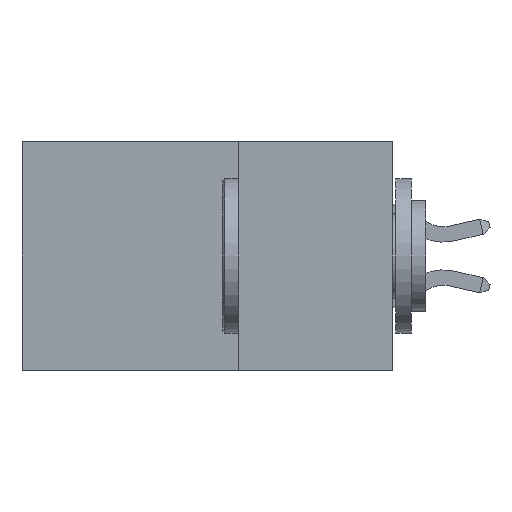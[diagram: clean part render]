
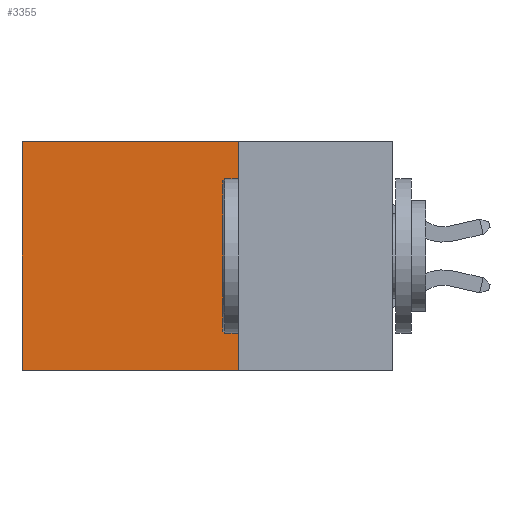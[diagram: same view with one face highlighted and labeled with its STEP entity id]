
A CAD part, left-side view. The second image highlights one B-rep face of the part: STEP entity #3355.
In plain terms, the highlighted planar face has unit normal (-1, 0, 0).
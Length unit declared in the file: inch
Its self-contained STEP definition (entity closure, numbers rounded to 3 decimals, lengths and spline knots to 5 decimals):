
#85 = CARTESIAN_POINT ( 'NONE',  ( 0.2875, 0.6, 0. ) ) ;
#1599 = DIRECTION ( 'NONE',  ( 0., 0., -1. ) ) ;
#1624 = DIRECTION ( 'NONE',  ( 1., 0., 0. ) ) ;
#1692 = CARTESIAN_POINT ( 'NONE',  ( 0.2875, 0.25, 0. ) ) ;
#2339 = VECTOR ( 'NONE', #8807, 39.37008 ) ;
#2370 = PLANE ( 'NONE',  #23709 ) ;
#3038 = LINE ( 'NONE', #85, #2339 ) ;
#3355 = ADVANCED_FACE ( 'NONE', ( #17948 ), #2370, .F. ) ;
#3544 = VERTEX_POINT ( 'NONE', #26406 ) ;
#4168 = EDGE_CURVE ( 'NONE', #6374, #3544, #4899, .T. ) ;
#4899 = LINE ( 'NONE', #24064, #10052 ) ;
#5327 = ORIENTED_EDGE ( 'NONE', *, *, #6823, .T. ) ;
#6047 = VERTEX_POINT ( 'NONE', #23977 ) ;
#6374 = VERTEX_POINT ( 'NONE', #18545 ) ;
#6777 = EDGE_CURVE ( 'NONE', #6047, #26854, #25365, .T. ) ;
#6823 = EDGE_CURVE ( 'NONE', #26854, #3544, #3038, .T. ) ;
#7695 = CARTESIAN_POINT ( 'NONE',  ( 0.2875, 0.25, 0. ) ) ;
#7789 = EDGE_CURVE ( 'NONE', #6047, #6374, #18022, .T. ) ;
#8807 = DIRECTION ( 'NONE',  ( 0., 0., -1. ) ) ;
#9910 = ORIENTED_EDGE ( 'NONE', *, *, #4168, .F. ) ;
#10052 = VECTOR ( 'NONE', #11175, 39.37008 ) ;
#10191 = ORIENTED_EDGE ( 'NONE', *, *, #7789, .F. ) ;
#11175 = DIRECTION ( 'NONE',  ( 0., 1., 0. ) ) ;
#17948 = FACE_OUTER_BOUND ( 'NONE', #20333, .T. ) ;
#18022 = LINE ( 'NONE', #7695, #21684 ) ;
#18545 = CARTESIAN_POINT ( 'NONE',  ( 0.2875, 0.25, -0.37 ) ) ;
#19340 = CARTESIAN_POINT ( 'NONE',  ( 0.2875, 0.6, 0. ) ) ;
#19705 = VECTOR ( 'NONE', #21659, 39.37008 ) ;
#19739 = ORIENTED_EDGE ( 'NONE', *, *, #6777, .T. ) ;
#20333 = EDGE_LOOP ( 'NONE', ( #5327, #9910, #10191, #19739 ) ) ;
#21659 = DIRECTION ( 'NONE',  ( 0., 1., 0. ) ) ;
#21684 = VECTOR ( 'NONE', #24963, 39.37008 ) ;
#23709 = AXIS2_PLACEMENT_3D ( 'NONE', #1692, #1624, #1599 ) ;
#23977 = CARTESIAN_POINT ( 'NONE',  ( 0.2875, 0.25, 0. ) ) ;
#24064 = CARTESIAN_POINT ( 'NONE',  ( 0.2875, 0.25, -0.37 ) ) ;
#24963 = DIRECTION ( 'NONE',  ( 0., 0., -1. ) ) ;
#25365 = LINE ( 'NONE', #25844, #19705 ) ;
#25844 = CARTESIAN_POINT ( 'NONE',  ( 0.2875, 0.25, 0. ) ) ;
#26406 = CARTESIAN_POINT ( 'NONE',  ( 0.2875, 0.6, -0.37 ) ) ;
#26854 = VERTEX_POINT ( 'NONE', #19340 ) ;
